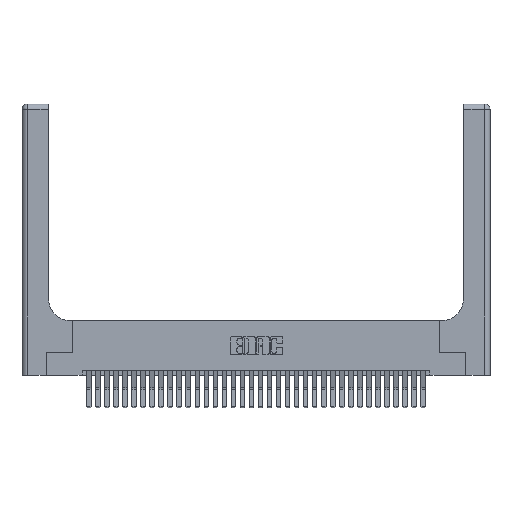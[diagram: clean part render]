
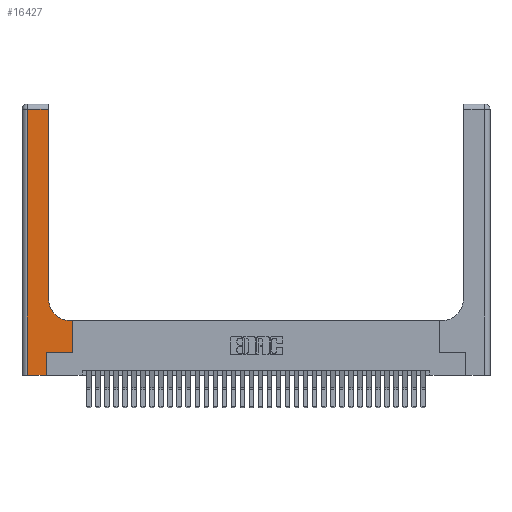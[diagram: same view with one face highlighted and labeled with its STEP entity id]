
A CAD part, top view. The second image highlights one B-rep face of the part: STEP entity #16427.
In plain terms, the highlighted planar face has unit normal (0, 0, 1).
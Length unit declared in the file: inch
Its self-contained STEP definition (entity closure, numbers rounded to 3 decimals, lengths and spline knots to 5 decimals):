
#852 = DIRECTION ( 'NONE',  ( 0., 1., 0. ) ) ;
#858 = AXIS2_PLACEMENT_3D ( 'NONE', #15197, #34387, #17953 ) ;
#887 = VECTOR ( 'NONE', #852, 39.37008 ) ;
#951 = CARTESIAN_POINT ( 'NONE',  ( 0.269, 0., 0.37 ) ) ;
#1659 = EDGE_CURVE ( 'NONE', #12302, #10381, #8241, .T. ) ;
#1711 = CARTESIAN_POINT ( 'NONE',  ( 0.5415, 0.85, 0.37 ) ) ;
#2682 = ORIENTED_EDGE ( 'NONE', *, *, #11389, .T. ) ;
#2847 = EDGE_CURVE ( 'NONE', #10381, #25451, #17656, .T. ) ;
#2901 = EDGE_CURVE ( 'NONE', #25451, #18808, #35249, .T. ) ;
#3630 = CARTESIAN_POINT ( 'NONE',  ( 0.269, 0., 0.37 ) ) ;
#4201 = CARTESIAN_POINT ( 'NONE',  ( 0., 2.94, 0.37 ) ) ;
#4472 = DIRECTION ( 'NONE',  ( 1., 0., 0. ) ) ;
#4554 = CARTESIAN_POINT ( 'NONE',  ( 0.269, 0.25, 0.37 ) ) ;
#4675 = AXIS2_PLACEMENT_3D ( 'NONE', #1711, #21002, #4472 ) ;
#5774 = CARTESIAN_POINT ( 'NONE',  ( 0.5585, 0.25, 0.37 ) ) ;
#5969 = CARTESIAN_POINT ( 'NONE',  ( 0.06, 2.94, 0.37 ) ) ;
#6127 = DIRECTION ( 'NONE',  ( 1., 0., 0. ) ) ;
#6201 = VECTOR ( 'NONE', #6127, 39.37008 ) ;
#6361 = ORIENTED_EDGE ( 'NONE', *, *, #33855, .T. ) ;
#6605 = ORIENTED_EDGE ( 'NONE', *, *, #2847, .T. ) ;
#8241 = LINE ( 'NONE', #3630, #887 ) ;
#9497 = CARTESIAN_POINT ( 'NONE',  ( 0.06, 0., 0.37 ) ) ;
#10084 = VECTOR ( 'NONE', #23207, 39.37008 ) ;
#10381 = VERTEX_POINT ( 'NONE', #18812 ) ;
#11340 = DIRECTION ( 'NONE',  ( 0., -1., 0. ) ) ;
#11389 = EDGE_CURVE ( 'NONE', #18808, #35638, #23865, .T. ) ;
#11821 = EDGE_CURVE ( 'NONE', #35638, #33687, #14016, .T. ) ;
#11946 = LINE ( 'NONE', #28427, #20133 ) ;
#12038 = ORIENTED_EDGE ( 'NONE', *, *, #11821, .T. ) ;
#12302 = VERTEX_POINT ( 'NONE', #951 ) ;
#12432 = DIRECTION ( 'NONE',  ( -1., 0., 0. ) ) ;
#13017 = DIRECTION ( 'NONE',  ( 0., 1., 0. ) ) ;
#13370 = ORIENTED_EDGE ( 'NONE', *, *, #14246, .T. ) ;
#13541 = LINE ( 'NONE', #25372, #6201 ) ;
#14016 = CIRCLE ( 'NONE', #4675, 0.25 ) ;
#14246 = EDGE_CURVE ( 'NONE', #34530, #22128, #20335, .T. ) ;
#15197 = CARTESIAN_POINT ( 'NONE',  ( 0., 3., 0.37 ) ) ;
#16236 = VECTOR ( 'NONE', #19449, 39.37008 ) ;
#16427 = ADVANCED_FACE ( 'NONE', ( #23602 ), #26096, .F. ) ;
#17387 = EDGE_CURVE ( 'NONE', #33687, #34530, #18815, .T. ) ;
#17656 = LINE ( 'NONE', #4554, #29655 ) ;
#17953 = DIRECTION ( 'NONE',  ( -1., 0., 0. ) ) ;
#18808 = VERTEX_POINT ( 'NONE', #24987 ) ;
#18812 = CARTESIAN_POINT ( 'NONE',  ( 0.269, 0.25, 0.37 ) ) ;
#18815 = LINE ( 'NONE', #30372, #16236 ) ;
#19449 = DIRECTION ( 'NONE',  ( 0., 1., 0. ) ) ;
#20133 = VECTOR ( 'NONE', #11340, 39.37008 ) ;
#20312 = EDGE_CURVE ( 'NONE', #34429, #12302, #13541, .T. ) ;
#20335 = LINE ( 'NONE', #4201, #34059 ) ;
#20651 = VECTOR ( 'NONE', #13017, 39.37008 ) ;
#21002 = DIRECTION ( 'NONE',  ( 0., 0., -1. ) ) ;
#21075 = DIRECTION ( 'NONE',  ( 1., 0., 0. ) ) ;
#22128 = VERTEX_POINT ( 'NONE', #5969 ) ;
#23207 = DIRECTION ( 'NONE',  ( -1., 0., 0. ) ) ;
#23602 = FACE_OUTER_BOUND ( 'NONE', #28391, .T. ) ;
#23865 = LINE ( 'NONE', #34228, #10084 ) ;
#24987 = CARTESIAN_POINT ( 'NONE',  ( 0.5585, 0.6, 0.37 ) ) ;
#25201 = ORIENTED_EDGE ( 'NONE', *, *, #1659, .T. ) ;
#25372 = CARTESIAN_POINT ( 'NONE',  ( 0., 0., 0.37 ) ) ;
#25451 = VERTEX_POINT ( 'NONE', #5774 ) ;
#26096 = PLANE ( 'NONE',  #858 ) ;
#26309 = CARTESIAN_POINT ( 'NONE',  ( 0.2915, 2.94, 0.37 ) ) ;
#26701 = CARTESIAN_POINT ( 'NONE',  ( 0.5585, 0.25, 0.37 ) ) ;
#28391 = EDGE_LOOP ( 'NONE', ( #34727, #13370, #6361, #34920, #25201, #6605, #34501, #2682, #12038 ) ) ;
#28427 = CARTESIAN_POINT ( 'NONE',  ( 0.06, 3., 0.37 ) ) ;
#29655 = VECTOR ( 'NONE', #21075, 39.37008 ) ;
#29984 = CARTESIAN_POINT ( 'NONE',  ( 0.2915, 0.85, 0.37 ) ) ;
#30372 = CARTESIAN_POINT ( 'NONE',  ( 0.2915, 3., 0.37 ) ) ;
#32345 = CARTESIAN_POINT ( 'NONE',  ( 0.5415, 0.6, 0.37 ) ) ;
#33687 = VERTEX_POINT ( 'NONE', #29984 ) ;
#33855 = EDGE_CURVE ( 'NONE', #22128, #34429, #11946, .T. ) ;
#34059 = VECTOR ( 'NONE', #12432, 39.37008 ) ;
#34228 = CARTESIAN_POINT ( 'NONE',  ( 0.2915, 0.6, 0.37 ) ) ;
#34387 = DIRECTION ( 'NONE',  ( 0., 0., -1. ) ) ;
#34429 = VERTEX_POINT ( 'NONE', #9497 ) ;
#34501 = ORIENTED_EDGE ( 'NONE', *, *, #2901, .T. ) ;
#34530 = VERTEX_POINT ( 'NONE', #26309 ) ;
#34727 = ORIENTED_EDGE ( 'NONE', *, *, #17387, .T. ) ;
#34920 = ORIENTED_EDGE ( 'NONE', *, *, #20312, .T. ) ;
#35249 = LINE ( 'NONE', #26701, #20651 ) ;
#35638 = VERTEX_POINT ( 'NONE', #32345 ) ;
